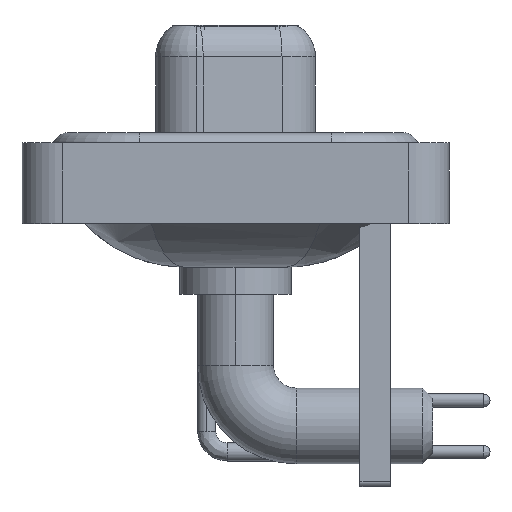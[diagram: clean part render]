
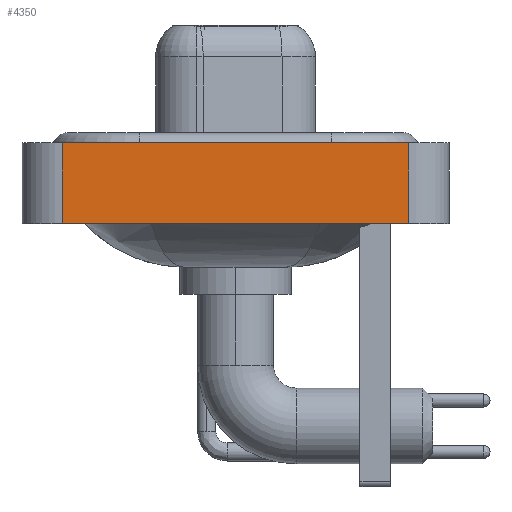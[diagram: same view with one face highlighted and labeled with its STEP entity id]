
A CAD part, left-side view. The second image highlights one B-rep face of the part: STEP entity #4350.
In plain terms, the highlighted planar face has unit normal (-1, 0, 0).
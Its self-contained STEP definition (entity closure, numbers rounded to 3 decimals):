
#718 = CARTESIAN_POINT ( 'NONE',  ( -7.3, -8.55, 0.4 ) ) ;
#852 = CARTESIAN_POINT ( 'NONE',  ( -7.3, 8.55, -3.6 ) ) ;
#2763 = VECTOR ( 'NONE', #10538, 1000. ) ;
#2842 = EDGE_CURVE ( 'NONE', #14874, #5947, #11678, .T. ) ;
#3734 = ORIENTED_EDGE ( 'NONE', *, *, #17875, .T. ) ;
#4350 = ADVANCED_FACE ( 'NONE', ( #11224 ), #7734, .T. ) ;
#4697 = EDGE_CURVE ( 'NONE', #5853, #20537, #18703, .T. ) ;
#5853 = VERTEX_POINT ( 'NONE', #10785 ) ;
#5947 = VERTEX_POINT ( 'NONE', #9254 ) ;
#7734 = PLANE ( 'NONE',  #21102 ) ;
#8243 = EDGE_LOOP ( 'NONE', ( #9101, #17433, #12604, #3734 ) ) ;
#9101 = ORIENTED_EDGE ( 'NONE', *, *, #2842, .T. ) ;
#9254 = CARTESIAN_POINT ( 'NONE',  ( -7.3, -8.55, 0.4 ) ) ;
#10538 = DIRECTION ( 'NONE',  ( 0., -1., 0. ) ) ;
#10785 = CARTESIAN_POINT ( 'NONE',  ( -7.3, 8.55, -3.6 ) ) ;
#10921 = CARTESIAN_POINT ( 'NONE',  ( -7.3, 8.55, 0.4 ) ) ;
#11224 = FACE_OUTER_BOUND ( 'NONE', #8243, .T. ) ;
#11678 = LINE ( 'NONE', #13524, #20018 ) ;
#12414 = DIRECTION ( 'NONE',  ( 0., 0., 1. ) ) ;
#12604 = ORIENTED_EDGE ( 'NONE', *, *, #4697, .F. ) ;
#13524 = CARTESIAN_POINT ( 'NONE',  ( -7.3, -8.55, -3.6 ) ) ;
#13787 = VECTOR ( 'NONE', #16588, 1000. ) ;
#14368 = DIRECTION ( 'NONE',  ( 0., 0., 1. ) ) ;
#14697 = DIRECTION ( 'NONE',  ( -1., 0., 0. ) ) ;
#14874 = VERTEX_POINT ( 'NONE', #16755 ) ;
#14934 = VECTOR ( 'NONE', #12414, 1000. ) ;
#14944 = DIRECTION ( 'NONE',  ( 0., 0., 1. ) ) ;
#16588 = DIRECTION ( 'NONE',  ( 0., -1., 0. ) ) ;
#16755 = CARTESIAN_POINT ( 'NONE',  ( -7.3, -8.55, -3.6 ) ) ;
#17433 = ORIENTED_EDGE ( 'NONE', *, *, #18776, .F. ) ;
#17875 = EDGE_CURVE ( 'NONE', #5853, #14874, #20141, .T. ) ;
#18703 = LINE ( 'NONE', #852, #14934 ) ;
#18776 = EDGE_CURVE ( 'NONE', #20537, #5947, #20811, .T. ) ;
#19361 = CARTESIAN_POINT ( 'NONE',  ( -7.3, -8.55, -3.6 ) ) ;
#20018 = VECTOR ( 'NONE', #14944, 1000. ) ;
#20141 = LINE ( 'NONE', #21334, #13787 ) ;
#20537 = VERTEX_POINT ( 'NONE', #10921 ) ;
#20811 = LINE ( 'NONE', #718, #2763 ) ;
#21102 = AXIS2_PLACEMENT_3D ( 'NONE', #19361, #14697, #14368 ) ;
#21334 = CARTESIAN_POINT ( 'NONE',  ( -7.3, -8.55, -3.6 ) ) ;
